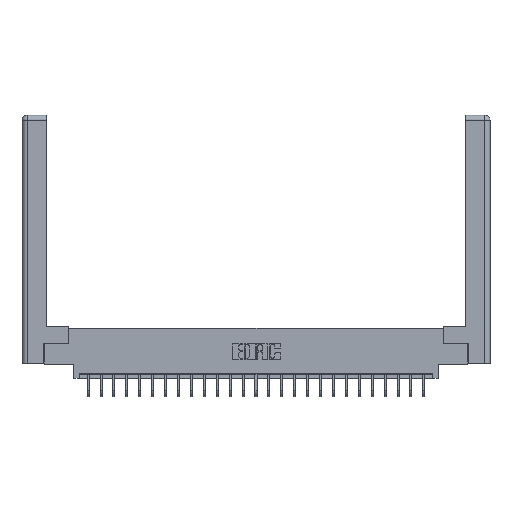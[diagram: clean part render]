
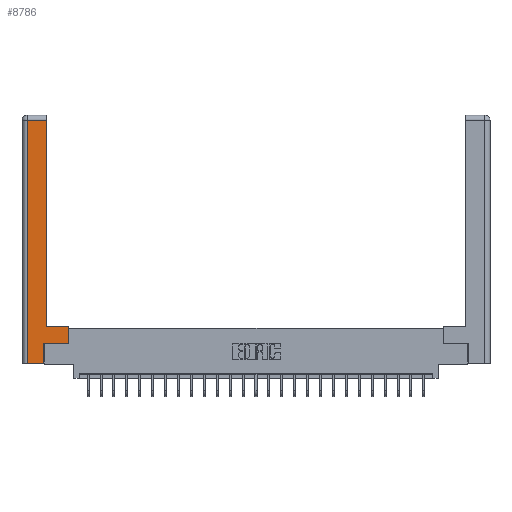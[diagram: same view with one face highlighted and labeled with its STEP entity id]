
A CAD part, top view. The second image highlights one B-rep face of the part: STEP entity #8786.
In plain terms, the highlighted planar face has unit normal (0, 0, 1).
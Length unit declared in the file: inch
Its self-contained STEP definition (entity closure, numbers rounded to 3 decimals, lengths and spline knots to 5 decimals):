
#917 = VECTOR ( 'NONE', #12868, 39.37008 ) ;
#1478 = CARTESIAN_POINT ( 'NONE',  ( 0.565, 0.45, 0. ) ) ;
#2260 = LINE ( 'NONE', #23384, #917 ) ;
#2333 = VECTOR ( 'NONE', #10877, 39.37008 ) ;
#2709 = ORIENTED_EDGE ( 'NONE', *, *, #16797, .T. ) ;
#3372 = ORIENTED_EDGE ( 'NONE', *, *, #9329, .T. ) ;
#3535 = ORIENTED_EDGE ( 'NONE', *, *, #22366, .T. ) ;
#4465 = LINE ( 'NONE', #25231, #17996 ) ;
#5565 = VECTOR ( 'NONE', #10871, 39.37008 ) ;
#5725 = DIRECTION ( 'NONE',  ( 0., -1., 0. ) ) ;
#5810 = EDGE_CURVE ( 'NONE', #11231, #18116, #4465, .T. ) ;
#5824 = DIRECTION ( 'NONE',  ( 0., 0., -1. ) ) ;
#6012 = LINE ( 'NONE', #11847, #15285 ) ;
#6389 = CARTESIAN_POINT ( 'NONE',  ( 0.265, 0., 0. ) ) ;
#7757 = ORIENTED_EDGE ( 'NONE', *, *, #18119, .T. ) ;
#7768 = CARTESIAN_POINT ( 'NONE',  ( 0.0615, 0., 0. ) ) ;
#8258 = VERTEX_POINT ( 'NONE', #24580 ) ;
#8467 = CARTESIAN_POINT ( 'NONE',  ( 0.565, 0.245, 0. ) ) ;
#8531 = VERTEX_POINT ( 'NONE', #21732 ) ;
#8786 = ADVANCED_FACE ( 'NONE', ( #9300 ), #16349, .F. ) ;
#9300 = FACE_OUTER_BOUND ( 'NONE', #19618, .T. ) ;
#9329 = EDGE_CURVE ( 'NONE', #20122, #21860, #20442, .T. ) ;
#9679 = EDGE_CURVE ( 'NONE', #16234, #20160, #6012, .T. ) ;
#10016 = VECTOR ( 'NONE', #19988, 39.37008 ) ;
#10871 = DIRECTION ( 'NONE',  ( 0., 1., 0. ) ) ;
#10877 = DIRECTION ( 'NONE',  ( 1., 0., 0. ) ) ;
#11192 = EDGE_CURVE ( 'NONE', #21860, #16234, #2260, .T. ) ;
#11231 = VERTEX_POINT ( 'NONE', #6389 ) ;
#11847 = CARTESIAN_POINT ( 'NONE',  ( 0.295, 3., 0. ) ) ;
#12002 = LINE ( 'NONE', #24399, #10016 ) ;
#12028 = CARTESIAN_POINT ( 'NONE',  ( 0., 0., 0. ) ) ;
#12868 = DIRECTION ( 'NONE',  ( -1., 0., 0. ) ) ;
#12911 = VECTOR ( 'NONE', #20246, 39.37008 ) ;
#14244 = ORIENTED_EDGE ( 'NONE', *, *, #11192, .T. ) ;
#14273 = LINE ( 'NONE', #7768, #23865 ) ;
#15285 = VECTOR ( 'NONE', #18364, 39.37008 ) ;
#15305 = CARTESIAN_POINT ( 'NONE',  ( 0.295, 2.94, 0. ) ) ;
#16234 = VERTEX_POINT ( 'NONE', #18003 ) ;
#16265 = DIRECTION ( 'NONE',  ( -1., 0., 0. ) ) ;
#16349 = PLANE ( 'NONE',  #16928 ) ;
#16797 = EDGE_CURVE ( 'NONE', #8258, #11231, #12002, .T. ) ;
#16928 = AXIS2_PLACEMENT_3D ( 'NONE', #12028, #5824, #16265 ) ;
#17996 = VECTOR ( 'NONE', #27375, 39.37008 ) ;
#18003 = CARTESIAN_POINT ( 'NONE',  ( 0.295, 0.45, 0. ) ) ;
#18116 = VERTEX_POINT ( 'NONE', #21178 ) ;
#18119 = EDGE_CURVE ( 'NONE', #18116, #20122, #24530, .T. ) ;
#18316 = CARTESIAN_POINT ( 'NONE',  ( 0.0615, 2.94, 0. ) ) ;
#18364 = DIRECTION ( 'NONE',  ( 0., 1., 0. ) ) ;
#18480 = LINE ( 'NONE', #18316, #12911 ) ;
#19607 = ORIENTED_EDGE ( 'NONE', *, *, #9679, .T. ) ;
#19618 = EDGE_LOOP ( 'NONE', ( #19607, #23396, #3535, #2709, #23770, #7757, #3372, #14244 ) ) ;
#19988 = DIRECTION ( 'NONE',  ( 1., 0., 0. ) ) ;
#20122 = VERTEX_POINT ( 'NONE', #25775 ) ;
#20160 = VERTEX_POINT ( 'NONE', #15305 ) ;
#20246 = DIRECTION ( 'NONE',  ( -1., 0., 0. ) ) ;
#20442 = LINE ( 'NONE', #21638, #5565 ) ;
#21178 = CARTESIAN_POINT ( 'NONE',  ( 0.265, 0.245, 0. ) ) ;
#21638 = CARTESIAN_POINT ( 'NONE',  ( 0.565, 0.45, 0. ) ) ;
#21732 = CARTESIAN_POINT ( 'NONE',  ( 0.0615, 2.94, 0. ) ) ;
#21860 = VERTEX_POINT ( 'NONE', #1478 ) ;
#22366 = EDGE_CURVE ( 'NONE', #8531, #8258, #14273, .T. ) ;
#22964 = EDGE_CURVE ( 'NONE', #20160, #8531, #18480, .T. ) ;
#23384 = CARTESIAN_POINT ( 'NONE',  ( 0.295, 0.45, 0. ) ) ;
#23396 = ORIENTED_EDGE ( 'NONE', *, *, #22964, .T. ) ;
#23770 = ORIENTED_EDGE ( 'NONE', *, *, #5810, .T. ) ;
#23865 = VECTOR ( 'NONE', #5725, 39.37008 ) ;
#24399 = CARTESIAN_POINT ( 'NONE',  ( 0.265, 0., 0. ) ) ;
#24530 = LINE ( 'NONE', #8467, #2333 ) ;
#24580 = CARTESIAN_POINT ( 'NONE',  ( 0.0615, 0., 0. ) ) ;
#25231 = CARTESIAN_POINT ( 'NONE',  ( 0.265, 0.245, 0. ) ) ;
#25775 = CARTESIAN_POINT ( 'NONE',  ( 0.565, 0.245, 0. ) ) ;
#27375 = DIRECTION ( 'NONE',  ( 0., 1., 0. ) ) ;
